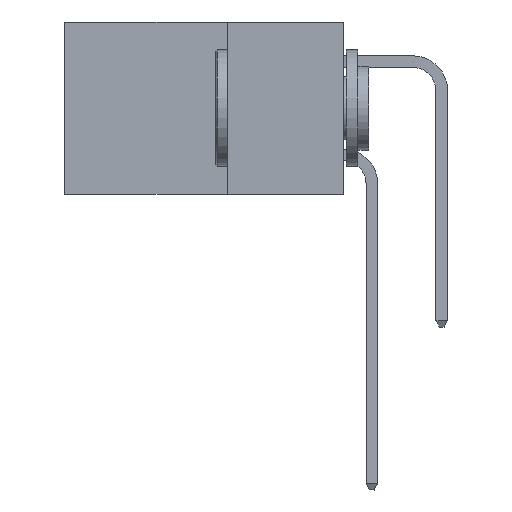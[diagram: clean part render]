
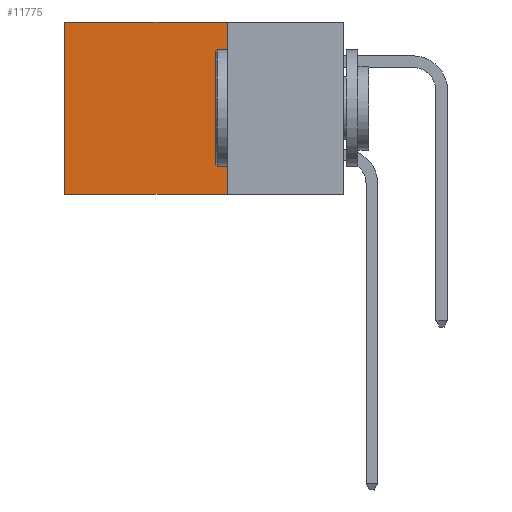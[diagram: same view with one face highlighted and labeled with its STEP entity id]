
A CAD part, left-side view. The second image highlights one B-rep face of the part: STEP entity #11775.
In plain terms, the highlighted planar face has unit normal (-1, 0, 0).
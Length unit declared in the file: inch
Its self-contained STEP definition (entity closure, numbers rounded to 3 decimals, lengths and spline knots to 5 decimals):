
#468 = ORIENTED_EDGE ( 'NONE', *, *, #892, .F. ) ;
#892 = EDGE_CURVE ( 'NONE', #12693, #9028, #1298, .T. ) ;
#955 = VERTEX_POINT ( 'NONE', #9574 ) ;
#1231 = DIRECTION ( 'NONE',  ( 1., 0., 0. ) ) ;
#1298 = LINE ( 'NONE', #13127, #16322 ) ;
#1442 = LINE ( 'NONE', #17283, #4810 ) ;
#3127 = CARTESIAN_POINT ( 'NONE',  ( 0.298, 0.6, 0. ) ) ;
#4231 = VECTOR ( 'NONE', #10314, 39.37008 ) ;
#4810 = VECTOR ( 'NONE', #12882, 39.37008 ) ;
#4853 = AXIS2_PLACEMENT_3D ( 'NONE', #9904, #1231, #11371 ) ;
#5598 = LINE ( 'NONE', #11766, #4231 ) ;
#5804 = CARTESIAN_POINT ( 'NONE',  ( 0.298, 0.25, 0. ) ) ;
#6953 = DIRECTION ( 'NONE',  ( 0., 0., -1. ) ) ;
#7601 = EDGE_CURVE ( 'NONE', #955, #16614, #5598, .T. ) ;
#7900 = ORIENTED_EDGE ( 'NONE', *, *, #13934, .T. ) ;
#8727 = VECTOR ( 'NONE', #6953, 39.37008 ) ;
#9028 = VERTEX_POINT ( 'NONE', #18426 ) ;
#9160 = EDGE_CURVE ( 'NONE', #955, #12693, #15591, .T. ) ;
#9574 = CARTESIAN_POINT ( 'NONE',  ( 0.298, 0.25, 0. ) ) ;
#9904 = CARTESIAN_POINT ( 'NONE',  ( 0.298, 0.25, 0. ) ) ;
#10314 = DIRECTION ( 'NONE',  ( 0., 1., 0. ) ) ;
#10964 = DIRECTION ( 'NONE',  ( 0., 1., 0. ) ) ;
#11371 = DIRECTION ( 'NONE',  ( 0., 0., -1. ) ) ;
#11766 = CARTESIAN_POINT ( 'NONE',  ( 0.298, 0.25, 0. ) ) ;
#11775 = ADVANCED_FACE ( 'NONE', ( #14480 ), #12776, .F. ) ;
#11777 = ORIENTED_EDGE ( 'NONE', *, *, #9160, .F. ) ;
#11782 = CARTESIAN_POINT ( 'NONE',  ( 0.298, 0.25, -0.37 ) ) ;
#12693 = VERTEX_POINT ( 'NONE', #11782 ) ;
#12760 = ORIENTED_EDGE ( 'NONE', *, *, #7601, .T. ) ;
#12776 = PLANE ( 'NONE',  #4853 ) ;
#12882 = DIRECTION ( 'NONE',  ( 0., 0., -1. ) ) ;
#13127 = CARTESIAN_POINT ( 'NONE',  ( 0.298, 0.25, -0.37 ) ) ;
#13934 = EDGE_CURVE ( 'NONE', #16614, #9028, #1442, .T. ) ;
#14480 = FACE_OUTER_BOUND ( 'NONE', #17537, .T. ) ;
#15591 = LINE ( 'NONE', #5804, #8727 ) ;
#16322 = VECTOR ( 'NONE', #10964, 39.37008 ) ;
#16614 = VERTEX_POINT ( 'NONE', #3127 ) ;
#17283 = CARTESIAN_POINT ( 'NONE',  ( 0.298, 0.6, 0. ) ) ;
#17537 = EDGE_LOOP ( 'NONE', ( #7900, #468, #11777, #12760 ) ) ;
#18426 = CARTESIAN_POINT ( 'NONE',  ( 0.298, 0.6, -0.37 ) ) ;
